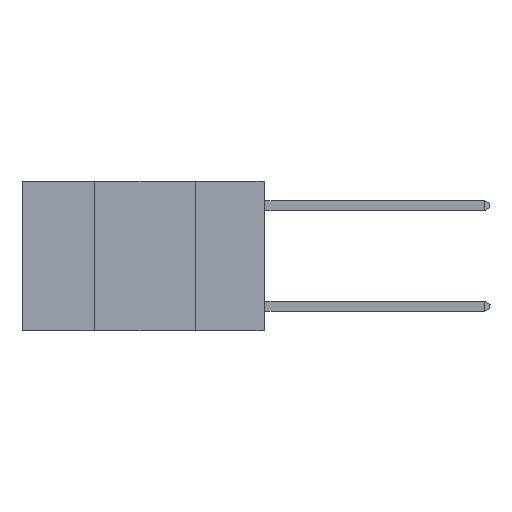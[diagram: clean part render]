
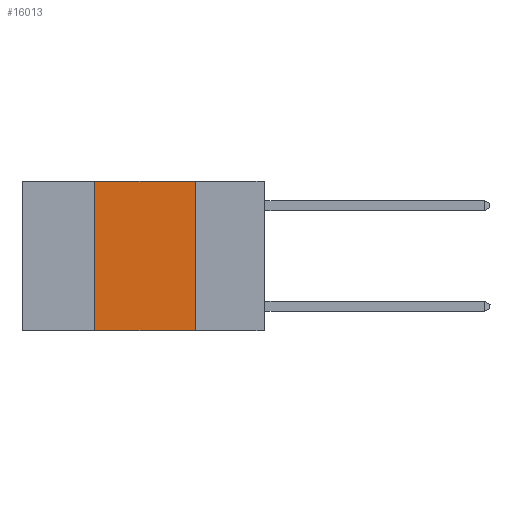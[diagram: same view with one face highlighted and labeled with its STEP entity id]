
A CAD part, left-side view. The second image highlights one B-rep face of the part: STEP entity #16013.
In plain terms, the highlighted planar face has unit normal (-1, 0, 0).
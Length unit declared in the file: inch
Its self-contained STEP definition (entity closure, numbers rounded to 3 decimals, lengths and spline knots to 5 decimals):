
#756 = LINE ( 'NONE', #13761, #23305 ) ;
#900 = EDGE_LOOP ( 'NONE', ( #11072, #23954, #15635, #28252 ) ) ;
#1541 = CARTESIAN_POINT ( 'NONE',  ( 0., 0.6, -0.37 ) ) ;
#2146 = VERTEX_POINT ( 'NONE', #22716 ) ;
#2677 = AXIS2_PLACEMENT_3D ( 'NONE', #7202, #18155, #5129 ) ;
#2918 = PLANE ( 'NONE',  #2677 ) ;
#3249 = VERTEX_POINT ( 'NONE', #17360 ) ;
#3775 = DIRECTION ( 'NONE',  ( 0., -1., 0. ) ) ;
#4999 = CARTESIAN_POINT ( 'NONE',  ( 0., 0.17, -0.37 ) ) ;
#5128 = EDGE_CURVE ( 'NONE', #14846, #2146, #25629, .T. ) ;
#5129 = DIRECTION ( 'NONE',  ( 0., 0., -1. ) ) ;
#6571 = EDGE_CURVE ( 'NONE', #14846, #6912, #12596, .T. ) ;
#6912 = VERTEX_POINT ( 'NONE', #4999 ) ;
#7202 = CARTESIAN_POINT ( 'NONE',  ( 0., 0.6, 0. ) ) ;
#7288 = DIRECTION ( 'NONE',  ( 0., 0., -1. ) ) ;
#7731 = CARTESIAN_POINT ( 'NONE',  ( 0., 0.42, -0.37 ) ) ;
#8261 = VECTOR ( 'NONE', #16998, 39.37008 ) ;
#8330 = CARTESIAN_POINT ( 'NONE',  ( 0., 0.42, 0. ) ) ;
#10748 = VECTOR ( 'NONE', #19882, 39.37008 ) ;
#10944 = EDGE_CURVE ( 'NONE', #3249, #6912, #756, .T. ) ;
#11072 = ORIENTED_EDGE ( 'NONE', *, *, #10944, .F. ) ;
#12596 = LINE ( 'NONE', #1541, #24184 ) ;
#13761 = CARTESIAN_POINT ( 'NONE',  ( 0., 0.17, 0. ) ) ;
#14846 = VERTEX_POINT ( 'NONE', #7731 ) ;
#15635 = ORIENTED_EDGE ( 'NONE', *, *, #5128, .F. ) ;
#16013 = ADVANCED_FACE ( 'NONE', ( #17027 ), #2918, .F. ) ;
#16998 = DIRECTION ( 'NONE',  ( 0., 0., 1. ) ) ;
#17027 = FACE_OUTER_BOUND ( 'NONE', #900, .T. ) ;
#17360 = CARTESIAN_POINT ( 'NONE',  ( 0., 0.17, 0. ) ) ;
#18155 = DIRECTION ( 'NONE',  ( 1., 0., 0. ) ) ;
#19882 = DIRECTION ( 'NONE',  ( 0., -1., 0. ) ) ;
#22716 = CARTESIAN_POINT ( 'NONE',  ( 0., 0.42, 0. ) ) ;
#22950 = EDGE_CURVE ( 'NONE', #2146, #3249, #28106, .T. ) ;
#23305 = VECTOR ( 'NONE', #7288, 39.37008 ) ;
#23954 = ORIENTED_EDGE ( 'NONE', *, *, #22950, .F. ) ;
#24184 = VECTOR ( 'NONE', #3775, 39.37008 ) ;
#25629 = LINE ( 'NONE', #8330, #8261 ) ;
#26346 = CARTESIAN_POINT ( 'NONE',  ( 0., 0.6, 0. ) ) ;
#28106 = LINE ( 'NONE', #26346, #10748 ) ;
#28252 = ORIENTED_EDGE ( 'NONE', *, *, #6571, .T. ) ;
